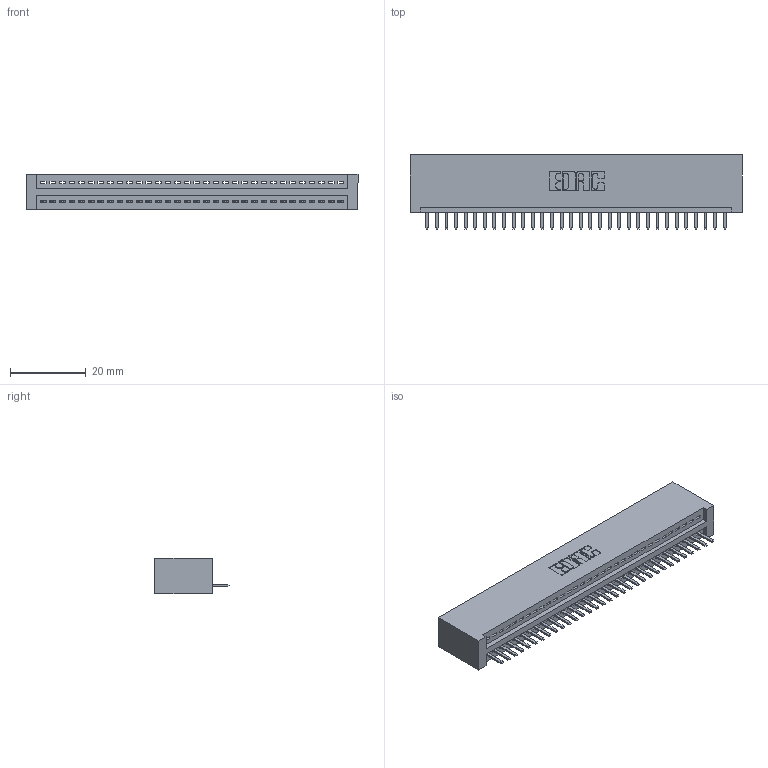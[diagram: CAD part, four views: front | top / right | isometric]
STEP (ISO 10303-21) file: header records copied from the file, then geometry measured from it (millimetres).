
FILE_DESCRIPTION (( 'STEP AP203' ), '1' );
FILE_NAME ('395-032-520-101.STEP', '2019-10-19T13:40:00', ( '' ), ( '' ), 'SwSTEP 2.0', 'SolidWorks 2016', '' );
FILE_SCHEMA (( 'CONFIG_CONTROL_DESIGN' ));
Length unit declared in the file: inch
Products named in the file (3): 395-032-520-101; 345 Part_No Mounting Lugs; 345-292-001_345-293-120
Assembly tree (33 placements, depth 2):
  395-032-520-101
    345 Part_No Mounting Lugs
    345-292-001_345-293-120  x32
Bounding box: 87.88 x 19.68 x 9.4 mm (x, y, z)
Volume: 8757.7 mm3; surface area: 11391.3 mm2
Topology: 33 solids, 33 shells, 2102 faces, 6205 edges, 4050 vertices
Faces by surface type: plane 1420, cylinder 682
Entity records: 25267 total; most frequent: CARTESIAN_POINT 4396, ORIENTED_EDGE 4350, DIRECTION 3835, EDGE_CURVE 2175, LINE 1919, VECTOR 1919, VERTEX_POINT 1446, AXIS2_PLACEMENT_3D 958
